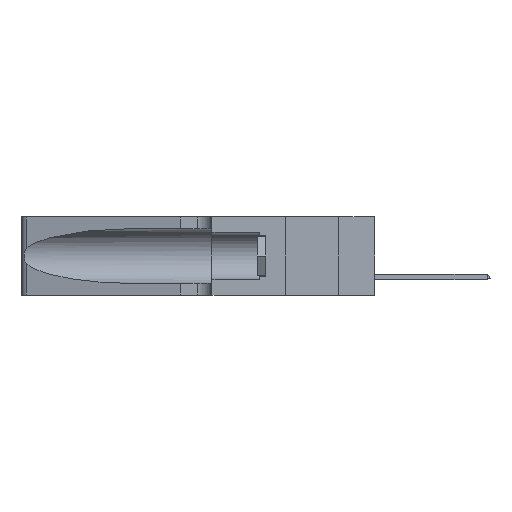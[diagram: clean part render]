
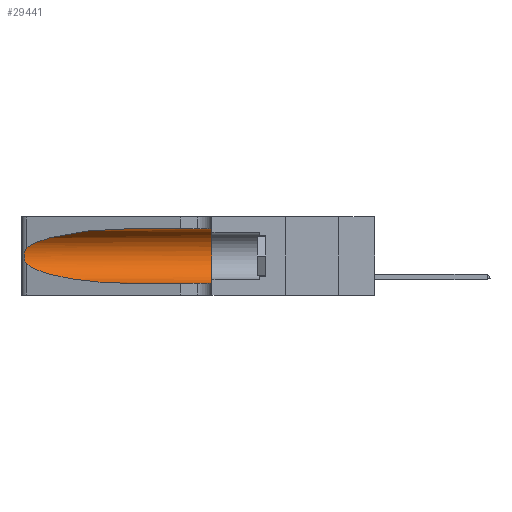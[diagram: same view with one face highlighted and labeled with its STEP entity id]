
A CAD part, left-side view. The second image highlights one B-rep face of the part: STEP entity #29441.
In plain terms, the highlighted cylindrical face has radius 3.308 mm (diameter 6.617 mm), a partial arc.
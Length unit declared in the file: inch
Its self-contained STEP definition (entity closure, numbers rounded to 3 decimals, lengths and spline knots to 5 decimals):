
#381 = CARTESIAN_POINT ( 'NONE',  ( 0.1305, 0.35, 0.31525 ) ) ;
#2164 = CARTESIAN_POINT ( 'NONE',  ( 0.1305, 1.61858, 0.31525 ) ) ;
#3178 = CARTESIAN_POINT ( 'NONE',  ( 0.25854, 1.2359, 0.20912 ) ) ;
#3213 = VERTEX_POINT ( 'NONE', #30954 ) ;
#4214 = CARTESIAN_POINT ( 'NONE',  ( 0.25487, 1.22718, 0.14631 ) ) ;
#5137 = VECTOR ( 'NONE', #9458, 39.37008 ) ;
#6605 = CARTESIAN_POINT ( 'NONE',  ( 0.1305, 0.35, 0.185 ) ) ;
#6875 = CARTESIAN_POINT ( 'NONE',  ( 0.1305, 0.72297, 0.05475 ) ) ;
#6909 = CARTESIAN_POINT ( 'NONE',  ( 0.2373, 1.15595, 0.28018 ) ) ;
#7153 = CARTESIAN_POINT ( 'NONE',  ( 0.18966, 0.96281, 0.31525 ) ) ;
#7636 = CARTESIAN_POINT ( 'NONE',  ( 0.1305, 0.72297, 0.05475 ) ) ;
#7879 = CARTESIAN_POINT ( 'NONE',  ( 0.26075, 1.23896, 0.19203 ) ) ;
#8241 =( BOUNDED_CURVE ( )  B_SPLINE_CURVE ( 3, ( #4214, #23386, #12909, #6875 ),
 .UNSPECIFIED., .F., .T. ) 
 B_SPLINE_CURVE_WITH_KNOTS ( ( 4, 4 ),
 ( 3.44316, 4.71239 ),
 .UNSPECIFIED. ) 
 CURVE ( )  GEOMETRIC_REPRESENTATION_ITEM ( )  RATIONAL_B_SPLINE_CURVE ( ( 1., 0.87, 0.87, 1. ) ) 
 REPRESENTATION_ITEM ( '' )  );
#8435 = CARTESIAN_POINT ( 'NONE',  ( 0.26017, 1.23833, 0.17102 ) ) ;
#8544 = CARTESIAN_POINT ( 'NONE',  ( 0.25555, 1.22993, 0.14849 ) ) ;
#8596 = EDGE_LOOP ( 'NONE', ( #20499, #25646, #32945, #24817, #34078, #10694 ) ) ;
#9458 = DIRECTION ( 'NONE',  ( 0., -1., 0. ) ) ;
#10694 = ORIENTED_EDGE ( 'NONE', *, *, #21656, .F. ) ;
#11384 = CARTESIAN_POINT ( 'NONE',  ( 0.25787, 1.23484, 0.2124 ) ) ;
#11709 = CARTESIAN_POINT ( 'NONE',  ( 0.26018, 1.23835, 0.19895 ) ) ;
#12578 = CARTESIAN_POINT ( 'NONE',  ( 0.25487, 1.22718, 0.22369 ) ) ;
#12674 = DIRECTION ( 'NONE',  ( 0., 1., 0. ) ) ;
#12825 = AXIS2_PLACEMENT_3D ( 'NONE', #6605, #12674, #20746 ) ;
#12909 = CARTESIAN_POINT ( 'NONE',  ( 0.18966, 0.96281, 0.05475 ) ) ;
#13861 = CARTESIAN_POINT ( 'NONE',  ( 0.1305, 0.35, 0.05475 ) ) ;
#14886 = FACE_OUTER_BOUND ( 'NONE', #8596, .T. ) ;
#14895 = CARTESIAN_POINT ( 'NONE',  ( 0.1305, 1.61858, 0.05475 ) ) ;
#16007 = VERTEX_POINT ( 'NONE', #13861 ) ;
#16218 = VECTOR ( 'NONE', #24216, 39.37008 ) ;
#16501 = CARTESIAN_POINT ( 'NONE',  ( 0.25487, 1.22718, 0.14631 ) ) ;
#16717 = CARTESIAN_POINT ( 'NONE',  ( 0.25789, 1.23486, 0.15765 ) ) ;
#16718 = VERTEX_POINT ( 'NONE', #35275 ) ;
#16977 = VERTEX_POINT ( 'NONE', #16994 ) ;
#16994 = CARTESIAN_POINT ( 'NONE',  ( 0.1305, 0.72297, 0.31525 ) ) ;
#17883 = CARTESIAN_POINT ( 'NONE',  ( 0.1305, 0.72297, 0.31525 ) ) ;
#18849 = EDGE_CURVE ( 'NONE', #16977, #16718, #19939, .T. ) ;
#19939 =( BOUNDED_CURVE ( )  B_SPLINE_CURVE ( 3, ( #17883, #7153, #6909, #12578 ),
 .UNSPECIFIED., .F., .T. ) 
 B_SPLINE_CURVE_WITH_KNOTS ( ( 4, 4 ),
 ( 1.5708, 2.84003 ),
 .UNSPECIFIED. ) 
 CURVE ( )  GEOMETRIC_REPRESENTATION_ITEM ( )  RATIONAL_B_SPLINE_CURVE ( ( 1., 0.87, 0.87, 1. ) ) 
 REPRESENTATION_ITEM ( '' )  );
#20499 = ORIENTED_EDGE ( 'NONE', *, *, #18849, .T. ) ;
#20746 = DIRECTION ( 'NONE',  ( 0., 0., 1. ) ) ;
#21524 = VERTEX_POINT ( 'NONE', #7636 ) ;
#21527 = LINE ( 'NONE', #14895, #5137 ) ;
#21656 = EDGE_CURVE ( 'NONE', #16977, #25367, #24435, .T. ) ;
#23005 = EDGE_CURVE ( 'NONE', #16718, #3213, #35059, .T. ) ;
#23386 = CARTESIAN_POINT ( 'NONE',  ( 0.2373, 1.15595, 0.08982 ) ) ;
#23521 = CIRCLE ( 'NONE', #12825, 0.13025 ) ;
#24216 = DIRECTION ( 'NONE',  ( 0., -1., 0. ) ) ;
#24240 = DIRECTION ( 'NONE',  ( 0., -1., 0. ) ) ;
#24435 = LINE ( 'NONE', #2164, #16218 ) ;
#24731 = CARTESIAN_POINT ( 'NONE',  ( 0.25639, 1.23186, 0.15144 ) ) ;
#24817 = ORIENTED_EDGE ( 'NONE', *, *, #28656, .T. ) ;
#24905 = EDGE_CURVE ( 'NONE', #25367, #16007, #23521, .T. ) ;
#25259 = CARTESIAN_POINT ( 'NONE',  ( 0.25639, 1.23184, 0.21858 ) ) ;
#25367 = VERTEX_POINT ( 'NONE', #381 ) ;
#25646 = ORIENTED_EDGE ( 'NONE', *, *, #23005, .T. ) ;
#26597 = CYLINDRICAL_SURFACE ( 'NONE', #33957, 0.13025 ) ;
#26928 = DIRECTION ( 'NONE',  ( 0., 0., -1. ) ) ;
#27620 = CARTESIAN_POINT ( 'NONE',  ( 0.26075, 1.23896, 0.178 ) ) ;
#27685 = CARTESIAN_POINT ( 'NONE',  ( 0.25555, 1.22994, 0.2215 ) ) ;
#28656 = EDGE_CURVE ( 'NONE', #21524, #16007, #21527, .T. ) ;
#29441 = ADVANCED_FACE ( 'NONE', ( #14886 ), #26597, .F. ) ;
#30954 = CARTESIAN_POINT ( 'NONE',  ( 0.25487, 1.22718, 0.14631 ) ) ;
#32899 = CARTESIAN_POINT ( 'NONE',  ( 0.25487, 1.22718, 0.22369 ) ) ;
#32920 = CARTESIAN_POINT ( 'NONE',  ( 0.1305, 1.61858, 0.185 ) ) ;
#32945 = ORIENTED_EDGE ( 'NONE', *, *, #35061, .T. ) ;
#33286 = CARTESIAN_POINT ( 'NONE',  ( 0.25856, 1.23593, 0.16098 ) ) ;
#33957 = AXIS2_PLACEMENT_3D ( 'NONE', #32920, #24240, #26928 ) ;
#34078 = ORIENTED_EDGE ( 'NONE', *, *, #24905, .F. ) ;
#35059 = B_SPLINE_CURVE_WITH_KNOTS ( 'NONE', 3,
 ( #32899, #27685, #25259, #11384, #3178, #11709, #7879, #27620, #8435, #33286, #16717, #24731, #8544, #16501 ),
 .UNSPECIFIED., .F., .F.,
 ( 4, 2, 2, 2, 2, 2, 4 ),
 ( 0., 0.00027, 0.00053, 0.00107, 0.0016, 0.00187, 0.00214 ),
 .UNSPECIFIED. ) ;
#35061 = EDGE_CURVE ( 'NONE', #3213, #21524, #8241, .T. ) ;
#35275 = CARTESIAN_POINT ( 'NONE',  ( 0.25487, 1.22718, 0.22369 ) ) ;
